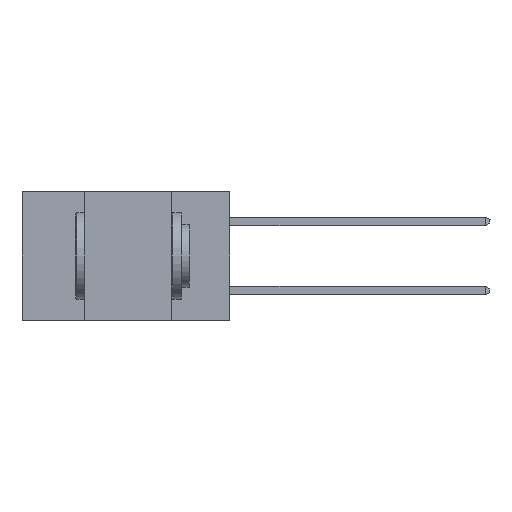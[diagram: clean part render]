
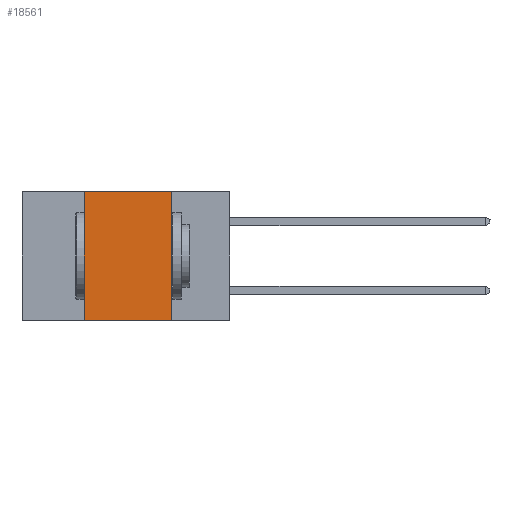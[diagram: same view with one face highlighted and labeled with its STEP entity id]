
A CAD part, left-side view. The second image highlights one B-rep face of the part: STEP entity #18561.
In plain terms, the highlighted planar face has unit normal (-1, 0, 0).
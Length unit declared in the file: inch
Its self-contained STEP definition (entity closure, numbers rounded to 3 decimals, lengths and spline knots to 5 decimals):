
#44 = CARTESIAN_POINT ( 'NONE',  ( 0., 0.6, 0. ) ) ;
#1480 = VECTOR ( 'NONE', #15421, 39.37008 ) ;
#1670 = PLANE ( 'NONE',  #15678 ) ;
#2461 = VERTEX_POINT ( 'NONE', #5952 ) ;
#3007 = DIRECTION ( 'NONE',  ( 0., 0., -1. ) ) ;
#4872 = ORIENTED_EDGE ( 'NONE', *, *, #9823, .T. ) ;
#4900 = CARTESIAN_POINT ( 'NONE',  ( 0., 0.17, 0. ) ) ;
#4903 = ORIENTED_EDGE ( 'NONE', *, *, #6572, .F. ) ;
#4927 = LINE ( 'NONE', #16623, #14263 ) ;
#5432 = CARTESIAN_POINT ( 'NONE',  ( 0., 0.42, 0. ) ) ;
#5784 = EDGE_CURVE ( 'NONE', #13871, #12664, #13322, .T. ) ;
#5885 = DIRECTION ( 'NONE',  ( 1., 0., 0. ) ) ;
#5938 = CARTESIAN_POINT ( 'NONE',  ( 0., 0.17, -0.37 ) ) ;
#5952 = CARTESIAN_POINT ( 'NONE',  ( 0., 0.42, -0.37 ) ) ;
#6023 = DIRECTION ( 'NONE',  ( 0., 0., -1. ) ) ;
#6056 = FACE_OUTER_BOUND ( 'NONE', #14594, .T. ) ;
#6572 = EDGE_CURVE ( 'NONE', #7949, #13871, #18469, .T. ) ;
#7949 = VERTEX_POINT ( 'NONE', #5432 ) ;
#8887 = LINE ( 'NONE', #17409, #12351 ) ;
#9823 = EDGE_CURVE ( 'NONE', #2461, #12664, #8887, .T. ) ;
#11729 = EDGE_CURVE ( 'NONE', #2461, #7949, #4927, .T. ) ;
#12076 = CARTESIAN_POINT ( 'NONE',  ( 0., 0.17, -0.37 ) ) ;
#12351 = VECTOR ( 'NONE', #16085, 39.37008 ) ;
#12664 = VERTEX_POINT ( 'NONE', #12076 ) ;
#13322 = LINE ( 'NONE', #5938, #16710 ) ;
#13871 = VERTEX_POINT ( 'NONE', #4900 ) ;
#14263 = VECTOR ( 'NONE', #15200, 39.37008 ) ;
#14594 = EDGE_LOOP ( 'NONE', ( #15121, #4903, #18538, #4872 ) ) ;
#15121 = ORIENTED_EDGE ( 'NONE', *, *, #5784, .F. ) ;
#15200 = DIRECTION ( 'NONE',  ( 0., 0., 1. ) ) ;
#15421 = DIRECTION ( 'NONE',  ( 0., -1., 0. ) ) ;
#15678 = AXIS2_PLACEMENT_3D ( 'NONE', #44, #5885, #3007 ) ;
#16085 = DIRECTION ( 'NONE',  ( 0., -1., 0. ) ) ;
#16623 = CARTESIAN_POINT ( 'NONE',  ( 0., 0.42, -0.37 ) ) ;
#16710 = VECTOR ( 'NONE', #6023, 39.37008 ) ;
#17409 = CARTESIAN_POINT ( 'NONE',  ( 0., 0.6, -0.37 ) ) ;
#18275 = CARTESIAN_POINT ( 'NONE',  ( 0., 0.6, 0. ) ) ;
#18469 = LINE ( 'NONE', #18275, #1480 ) ;
#18538 = ORIENTED_EDGE ( 'NONE', *, *, #11729, .F. ) ;
#18561 = ADVANCED_FACE ( 'NONE', ( #6056 ), #1670, .F. ) ;
